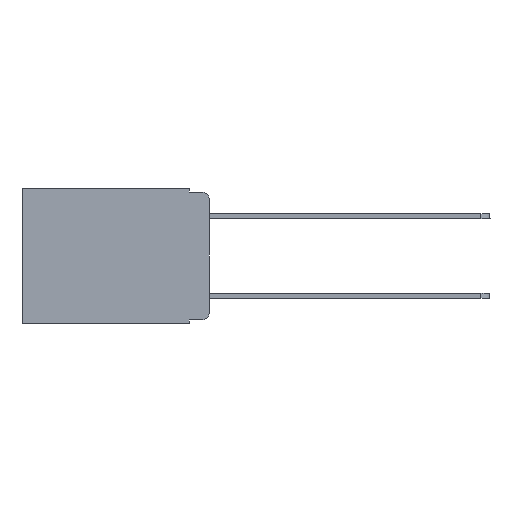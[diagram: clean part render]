
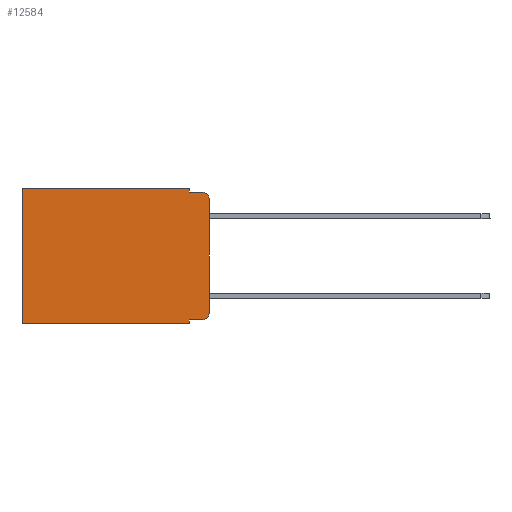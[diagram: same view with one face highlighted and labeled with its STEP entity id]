
A CAD part, left-side view. The second image highlights one B-rep face of the part: STEP entity #12584.
In plain terms, the highlighted planar face has unit normal (-1, 0, 0).
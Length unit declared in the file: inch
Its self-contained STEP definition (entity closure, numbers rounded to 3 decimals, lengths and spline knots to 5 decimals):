
#401 = DIRECTION ( 'NONE',  ( 0., -1., 0. ) ) ;
#459 = LINE ( 'NONE', #8343, #4455 ) ;
#804 = CARTESIAN_POINT ( 'NONE',  ( 0.298, 0.051, 0. ) ) ;
#995 = CARTESIAN_POINT ( 'NONE',  ( 0.298, 0., -0.03 ) ) ;
#1124 = FACE_OUTER_BOUND ( 'NONE', #5584, .T. ) ;
#1202 = LINE ( 'NONE', #15175, #21158 ) ;
#1805 = CARTESIAN_POINT ( 'NONE',  ( 0.298, 0.02, -0.03 ) ) ;
#1808 = ORIENTED_EDGE ( 'NONE', *, *, #13808, .T. ) ;
#2248 = ORIENTED_EDGE ( 'NONE', *, *, #10687, .F. ) ;
#2385 = CARTESIAN_POINT ( 'NONE',  ( 0.298, 0.02, -0.01 ) ) ;
#2418 = EDGE_CURVE ( 'NONE', #15926, #19096, #12187, .T. ) ;
#3240 = AXIS2_PLACEMENT_3D ( 'NONE', #1805, #13578, #9554 ) ;
#3248 = ORIENTED_EDGE ( 'NONE', *, *, #19850, .F. ) ;
#3412 = AXIS2_PLACEMENT_3D ( 'NONE', #14825, #20514, #17025 ) ;
#3732 = EDGE_CURVE ( 'NONE', #7471, #8193, #14613, .T. ) ;
#3975 = AXIS2_PLACEMENT_3D ( 'NONE', #16655, #24569, #22627 ) ;
#4133 = ORIENTED_EDGE ( 'NONE', *, *, #4393, .F. ) ;
#4393 = EDGE_CURVE ( 'NONE', #8193, #22831, #459, .T. ) ;
#4455 = VECTOR ( 'NONE', #6407, 39.37008 ) ;
#4509 = CARTESIAN_POINT ( 'NONE',  ( 0.298, 0.051, -0.343 ) ) ;
#4681 = VECTOR ( 'NONE', #401, 39.37008 ) ;
#5584 = EDGE_LOOP ( 'NONE', ( #7627, #13754, #4133, #6866, #15491, #1808, #2248, #3248, #22863, #24662 ) ) ;
#5761 = EDGE_CURVE ( 'NONE', #10168, #19096, #15819, .T. ) ;
#6407 = DIRECTION ( 'NONE',  ( 0., -1., 0. ) ) ;
#6626 = LINE ( 'NONE', #804, #13494 ) ;
#6819 = PLANE ( 'NONE',  #3975 ) ;
#6866 = ORIENTED_EDGE ( 'NONE', *, *, #3732, .F. ) ;
#7471 = VERTEX_POINT ( 'NONE', #18946 ) ;
#7627 = ORIENTED_EDGE ( 'NONE', *, *, #2418, .F. ) ;
#7766 = EDGE_CURVE ( 'NONE', #16267, #10168, #12313, .T. ) ;
#8165 = DIRECTION ( 'NONE',  ( 0., 0., -1. ) ) ;
#8193 = VERTEX_POINT ( 'NONE', #21868 ) ;
#8343 = CARTESIAN_POINT ( 'NONE',  ( 0.298, 0.051, -0.01 ) ) ;
#8417 = CARTESIAN_POINT ( 'NONE',  ( 0.298, 0., 0. ) ) ;
#8991 = VECTOR ( 'NONE', #23827, 39.37008 ) ;
#9080 = CARTESIAN_POINT ( 'NONE',  ( 0.298, 0.473, 0. ) ) ;
#9156 = DIRECTION ( 'NONE',  ( 0., 0., -1. ) ) ;
#9197 = VECTOR ( 'NONE', #8165, 39.37008 ) ;
#9554 = DIRECTION ( 'NONE',  ( 0., 0., -1. ) ) ;
#10168 = VERTEX_POINT ( 'NONE', #14838 ) ;
#10687 = EDGE_CURVE ( 'NONE', #15072, #17740, #17862, .T. ) ;
#12035 = DIRECTION ( 'NONE',  ( 0., 1., 0. ) ) ;
#12187 = LINE ( 'NONE', #8417, #9197 ) ;
#12313 = LINE ( 'NONE', #22286, #4681 ) ;
#12584 = ADVANCED_FACE ( 'NONE', ( #1124 ), #6819, .F. ) ;
#13494 = VECTOR ( 'NONE', #16457, 39.37008 ) ;
#13578 = DIRECTION ( 'NONE',  ( -1., 0., 0. ) ) ;
#13625 = CARTESIAN_POINT ( 'NONE',  ( 0.298, 0., -0.313 ) ) ;
#13739 = CARTESIAN_POINT ( 'NONE',  ( 0.298, 0.473, -0.343 ) ) ;
#13754 = ORIENTED_EDGE ( 'NONE', *, *, #21848, .T. ) ;
#13808 = EDGE_CURVE ( 'NONE', #16318, #17740, #20288, .T. ) ;
#14382 = CIRCLE ( 'NONE', #3240, 0.02 ) ;
#14613 = LINE ( 'NONE', #15133, #24748 ) ;
#14825 = CARTESIAN_POINT ( 'NONE',  ( 0.298, 0.02, -0.313 ) ) ;
#14838 = CARTESIAN_POINT ( 'NONE',  ( 0.298, 0.02, -0.333 ) ) ;
#15072 = VERTEX_POINT ( 'NONE', #4509 ) ;
#15133 = CARTESIAN_POINT ( 'NONE',  ( 0.298, 0.051, 0. ) ) ;
#15175 = CARTESIAN_POINT ( 'NONE',  ( 0.298, 0., 0. ) ) ;
#15491 = ORIENTED_EDGE ( 'NONE', *, *, #24940, .T. ) ;
#15819 = CIRCLE ( 'NONE', #3412, 0.02 ) ;
#15926 = VERTEX_POINT ( 'NONE', #995 ) ;
#16267 = VERTEX_POINT ( 'NONE', #16748 ) ;
#16318 = VERTEX_POINT ( 'NONE', #9080 ) ;
#16457 = DIRECTION ( 'NONE',  ( 0., 0., -1. ) ) ;
#16655 = CARTESIAN_POINT ( 'NONE',  ( 0.298, 0., 0. ) ) ;
#16748 = CARTESIAN_POINT ( 'NONE',  ( 0.298, 0.051, -0.333 ) ) ;
#17025 = DIRECTION ( 'NONE',  ( 0., 0., -1. ) ) ;
#17740 = VERTEX_POINT ( 'NONE', #13739 ) ;
#17862 = LINE ( 'NONE', #23819, #25073 ) ;
#18946 = CARTESIAN_POINT ( 'NONE',  ( 0.298, 0.051, 0. ) ) ;
#19096 = VERTEX_POINT ( 'NONE', #13625 ) ;
#19850 = EDGE_CURVE ( 'NONE', #16267, #15072, #6626, .T. ) ;
#20288 = LINE ( 'NONE', #21752, #8991 ) ;
#20514 = DIRECTION ( 'NONE',  ( -1., 0., 0. ) ) ;
#21008 = DIRECTION ( 'NONE',  ( 0., 1., 0. ) ) ;
#21158 = VECTOR ( 'NONE', #21008, 39.37008 ) ;
#21752 = CARTESIAN_POINT ( 'NONE',  ( 0.298, 0.473, 0. ) ) ;
#21848 = EDGE_CURVE ( 'NONE', #15926, #22831, #14382, .T. ) ;
#21868 = CARTESIAN_POINT ( 'NONE',  ( 0.298, 0.051, -0.01 ) ) ;
#22286 = CARTESIAN_POINT ( 'NONE',  ( 0.298, 0.051, -0.333 ) ) ;
#22627 = DIRECTION ( 'NONE',  ( 0., 0., -1. ) ) ;
#22831 = VERTEX_POINT ( 'NONE', #2385 ) ;
#22863 = ORIENTED_EDGE ( 'NONE', *, *, #7766, .T. ) ;
#23819 = CARTESIAN_POINT ( 'NONE',  ( 0.298, 0., -0.343 ) ) ;
#23827 = DIRECTION ( 'NONE',  ( 0., 0., -1. ) ) ;
#24569 = DIRECTION ( 'NONE',  ( 1., 0., 0. ) ) ;
#24662 = ORIENTED_EDGE ( 'NONE', *, *, #5761, .T. ) ;
#24748 = VECTOR ( 'NONE', #9156, 39.37008 ) ;
#24940 = EDGE_CURVE ( 'NONE', #7471, #16318, #1202, .T. ) ;
#25073 = VECTOR ( 'NONE', #12035, 39.37008 ) ;
